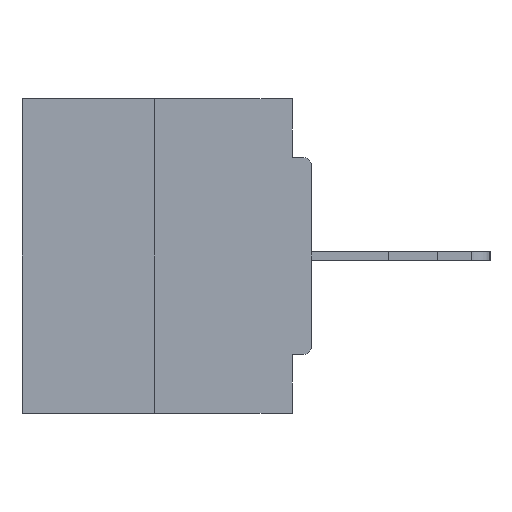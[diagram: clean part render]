
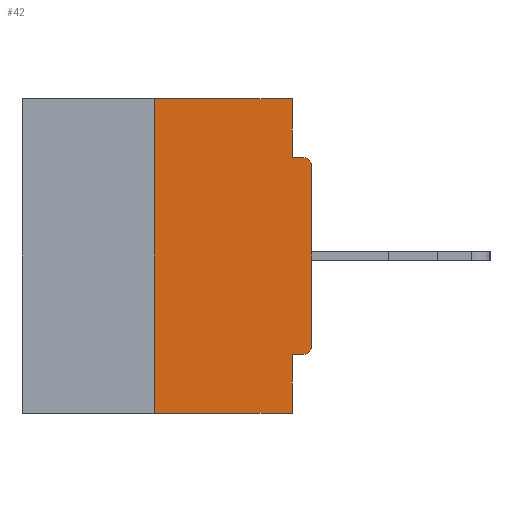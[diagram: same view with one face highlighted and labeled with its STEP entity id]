
A CAD part, left-side view. The second image highlights one B-rep face of the part: STEP entity #42.
In plain terms, the highlighted planar face has unit normal (-1, 0, 0).
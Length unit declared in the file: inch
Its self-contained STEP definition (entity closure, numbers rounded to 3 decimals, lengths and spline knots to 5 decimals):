
#42 = ADVANCED_FACE ( 'NONE', ( #36397 ), #26966, .F. ) ;
#401 = CARTESIAN_POINT ( 'NONE',  ( 0., 0.25, -0.5 ) ) ;
#625 = DIRECTION ( 'NONE',  ( 0., -1., 0. ) ) ;
#1262 = ORIENTED_EDGE ( 'NONE', *, *, #30627, .T. ) ;
#1368 = DIRECTION ( 'NONE',  ( -1., 0., 0. ) ) ;
#1375 = EDGE_CURVE ( 'NONE', #2408, #2082, #15232, .T. ) ;
#2082 = VERTEX_POINT ( 'NONE', #24671 ) ;
#2408 = VERTEX_POINT ( 'NONE', #21782 ) ;
#2412 = EDGE_LOOP ( 'NONE', ( #7379, #6467, #29622, #35598, #37979, #5081, #1262, #36964, #18661, #15920 ) ) ;
#2638 = DIRECTION ( 'NONE',  ( 0., 0., -1. ) ) ;
#2735 = VECTOR ( 'NONE', #19462, 39.37008 ) ;
#3804 = CARTESIAN_POINT ( 'NONE',  ( 0., 0.46, 0. ) ) ;
#3851 = CARTESIAN_POINT ( 'NONE',  ( 0., 0., 0. ) ) ;
#4607 = LINE ( 'NONE', #36215, #34319 ) ;
#5081 = ORIENTED_EDGE ( 'NONE', *, *, #1375, .T. ) ;
#5282 = CARTESIAN_POINT ( 'NONE',  ( 0., 0.031, -0.0935 ) ) ;
#5687 = VERTEX_POINT ( 'NONE', #5282 ) ;
#6017 = VECTOR ( 'NONE', #12808, 39.37008 ) ;
#6160 = VECTOR ( 'NONE', #33028, 39.37008 ) ;
#6189 = CARTESIAN_POINT ( 'NONE',  ( 0., 0.015, -0.0935 ) ) ;
#6467 = ORIENTED_EDGE ( 'NONE', *, *, #36355, .F. ) ;
#6737 = DIRECTION ( 'NONE',  ( 0., 0., 1. ) ) ;
#7260 = VECTOR ( 'NONE', #25158, 39.37008 ) ;
#7379 = ORIENTED_EDGE ( 'NONE', *, *, #25612, .F. ) ;
#7465 = CARTESIAN_POINT ( 'NONE',  ( 0., 0.25, 0. ) ) ;
#8381 = VECTOR ( 'NONE', #6737, 39.37008 ) ;
#9223 = CARTESIAN_POINT ( 'NONE',  ( 0., 0.031, -0.4065 ) ) ;
#9326 = LINE ( 'NONE', #3851, #8381 ) ;
#9349 = CARTESIAN_POINT ( 'NONE',  ( 0., 0.031, -0.5 ) ) ;
#11932 = VERTEX_POINT ( 'NONE', #9223 ) ;
#12808 = DIRECTION ( 'NONE',  ( 0., -1., 0. ) ) ;
#15003 = VECTOR ( 'NONE', #17842, 39.37008 ) ;
#15065 = LINE ( 'NONE', #9349, #6160 ) ;
#15232 = CIRCLE ( 'NONE', #23479, 0.015 ) ;
#15920 = ORIENTED_EDGE ( 'NONE', *, *, #25551, .F. ) ;
#16932 = VERTEX_POINT ( 'NONE', #401 ) ;
#17842 = DIRECTION ( 'NONE',  ( 0., -1., 0. ) ) ;
#18661 = ORIENTED_EDGE ( 'NONE', *, *, #26472, .F. ) ;
#18677 = LINE ( 'NONE', #7465, #2735 ) ;
#19307 = CARTESIAN_POINT ( 'NONE',  ( 0., 0.015, -0.1085 ) ) ;
#19462 = DIRECTION ( 'NONE',  ( 0., 0., 1. ) ) ;
#21782 = CARTESIAN_POINT ( 'NONE',  ( 0., 0.015, -0.4065 ) ) ;
#22177 = CARTESIAN_POINT ( 'NONE',  ( 0., 0., -0.4065 ) ) ;
#22205 = VERTEX_POINT ( 'NONE', #38503 ) ;
#22249 = VERTEX_POINT ( 'NONE', #32963 ) ;
#22322 = DIRECTION ( 'NONE',  ( 0., 0., -1. ) ) ;
#22466 = AXIS2_PLACEMENT_3D ( 'NONE', #3804, #30794, #34127 ) ;
#23443 = EDGE_CURVE ( 'NONE', #16932, #32719, #4607, .T. ) ;
#23479 = AXIS2_PLACEMENT_3D ( 'NONE', #28514, #34036, #33931 ) ;
#24671 = CARTESIAN_POINT ( 'NONE',  ( 0., 0., -0.3915 ) ) ;
#24802 = VECTOR ( 'NONE', #2638, 39.37008 ) ;
#25158 = DIRECTION ( 'NONE',  ( 0., 1., 0. ) ) ;
#25551 = EDGE_CURVE ( 'NONE', #22249, #5687, #32605, .T. ) ;
#25612 = EDGE_CURVE ( 'NONE', #36250, #22249, #30772, .T. ) ;
#26472 = EDGE_CURVE ( 'NONE', #5687, #34160, #37584, .T. ) ;
#26966 = PLANE ( 'NONE',  #22466 ) ;
#27559 = EDGE_CURVE ( 'NONE', #22205, #34160, #35205, .T. ) ;
#27638 = CARTESIAN_POINT ( 'NONE',  ( 0., 0., -0.0935 ) ) ;
#28514 = CARTESIAN_POINT ( 'NONE',  ( 0., 0.015, -0.3915 ) ) ;
#29229 = CARTESIAN_POINT ( 'NONE',  ( 0., 0.031, 0. ) ) ;
#29400 = EDGE_CURVE ( 'NONE', #2408, #11932, #30982, .T. ) ;
#29622 = ORIENTED_EDGE ( 'NONE', *, *, #23443, .T. ) ;
#30627 = EDGE_CURVE ( 'NONE', #2082, #22205, #9326, .T. ) ;
#30772 = LINE ( 'NONE', #32558, #15003 ) ;
#30794 = DIRECTION ( 'NONE',  ( 1., 0., 0. ) ) ;
#30845 = CARTESIAN_POINT ( 'NONE',  ( 0., 0.25, 0. ) ) ;
#30982 = LINE ( 'NONE', #22177, #7260 ) ;
#32558 = CARTESIAN_POINT ( 'NONE',  ( 0., 0.46, 0. ) ) ;
#32605 = LINE ( 'NONE', #29229, #24802 ) ;
#32719 = VERTEX_POINT ( 'NONE', #37311 ) ;
#32963 = CARTESIAN_POINT ( 'NONE',  ( 0., 0.031, 0. ) ) ;
#33028 = DIRECTION ( 'NONE',  ( 0., 0., -1. ) ) ;
#33931 = DIRECTION ( 'NONE',  ( 0., 0., -1. ) ) ;
#34036 = DIRECTION ( 'NONE',  ( -1., 0., 0. ) ) ;
#34127 = DIRECTION ( 'NONE',  ( 0., 0., -1. ) ) ;
#34160 = VERTEX_POINT ( 'NONE', #6189 ) ;
#34205 = AXIS2_PLACEMENT_3D ( 'NONE', #19307, #1368, #22322 ) ;
#34319 = VECTOR ( 'NONE', #625, 39.37008 ) ;
#34767 = EDGE_CURVE ( 'NONE', #11932, #32719, #15065, .T. ) ;
#35205 = CIRCLE ( 'NONE', #34205, 0.015 ) ;
#35598 = ORIENTED_EDGE ( 'NONE', *, *, #34767, .F. ) ;
#36215 = CARTESIAN_POINT ( 'NONE',  ( 0., 0.46, -0.5 ) ) ;
#36250 = VERTEX_POINT ( 'NONE', #30845 ) ;
#36355 = EDGE_CURVE ( 'NONE', #16932, #36250, #18677, .T. ) ;
#36397 = FACE_OUTER_BOUND ( 'NONE', #2412, .T. ) ;
#36964 = ORIENTED_EDGE ( 'NONE', *, *, #27559, .T. ) ;
#37311 = CARTESIAN_POINT ( 'NONE',  ( 0., 0.031, -0.5 ) ) ;
#37584 = LINE ( 'NONE', #27638, #6017 ) ;
#37979 = ORIENTED_EDGE ( 'NONE', *, *, #29400, .F. ) ;
#38503 = CARTESIAN_POINT ( 'NONE',  ( 0., 0., -0.1085 ) ) ;
